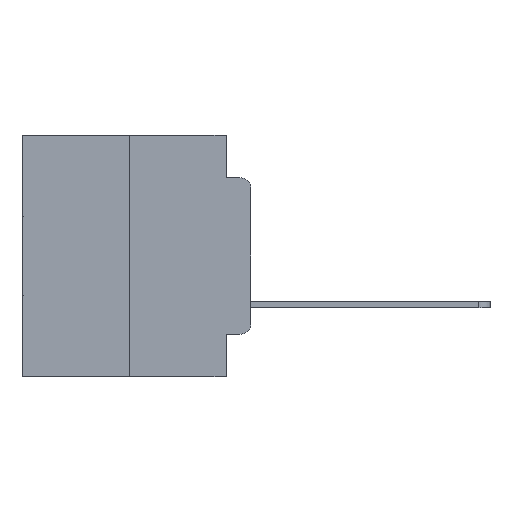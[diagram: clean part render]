
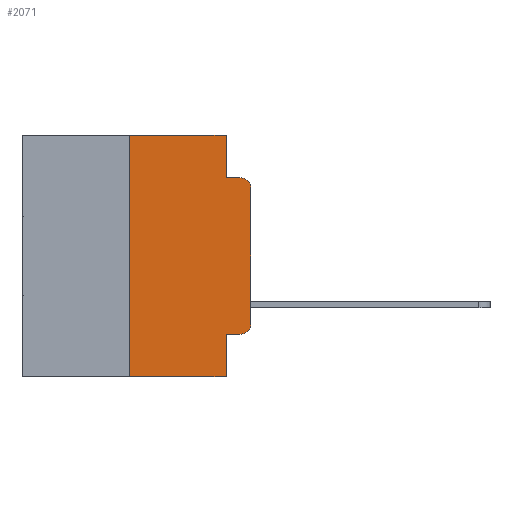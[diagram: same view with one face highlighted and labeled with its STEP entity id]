
A CAD part, left-side view. The second image highlights one B-rep face of the part: STEP entity #2071.
In plain terms, the highlighted planar face has unit normal (-1, 0, 0).
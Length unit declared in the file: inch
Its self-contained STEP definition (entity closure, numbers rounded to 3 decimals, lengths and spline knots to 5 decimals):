
#182 = DIRECTION ( 'NONE',  ( 0., 0., -1. ) ) ;
#361 = VECTOR ( 'NONE', #6799, 39.37008 ) ;
#924 = LINE ( 'NONE', #29368, #7049 ) ;
#1995 = VECTOR ( 'NONE', #3544, 39.37008 ) ;
#2071 = ADVANCED_FACE ( 'NONE', ( #7758 ), #21484, .F. ) ;
#2666 = VERTEX_POINT ( 'NONE', #7861 ) ;
#2777 = ORIENTED_EDGE ( 'NONE', *, *, #12554, .T. ) ;
#2829 = LINE ( 'NONE', #22086, #1995 ) ;
#3054 = VERTEX_POINT ( 'NONE', #5942 ) ;
#3544 = DIRECTION ( 'NONE',  ( 0., 0., -1. ) ) ;
#3761 = VERTEX_POINT ( 'NONE', #12208 ) ;
#4199 = CARTESIAN_POINT ( 'NONE',  ( 0., 0.051, -0.0885 ) ) ;
#4955 = DIRECTION ( 'NONE',  ( -1., 0., 0. ) ) ;
#5606 = ORIENTED_EDGE ( 'NONE', *, *, #14375, .T. ) ;
#5942 = CARTESIAN_POINT ( 'NONE',  ( 0., 0.02, -0.4115 ) ) ;
#6031 = AXIS2_PLACEMENT_3D ( 'NONE', #27563, #15197, #182 ) ;
#6092 = DIRECTION ( 'NONE',  ( 0., -1., 0. ) ) ;
#6799 = DIRECTION ( 'NONE',  ( 0., -1., 0. ) ) ;
#7049 = VECTOR ( 'NONE', #14979, 39.37008 ) ;
#7201 = ORIENTED_EDGE ( 'NONE', *, *, #12642, .F. ) ;
#7606 = VECTOR ( 'NONE', #6092, 39.37008 ) ;
#7656 = CARTESIAN_POINT ( 'NONE',  ( 0., 0., -0.3915 ) ) ;
#7758 = FACE_OUTER_BOUND ( 'NONE', #16010, .T. ) ;
#7861 = CARTESIAN_POINT ( 'NONE',  ( 0., 0.051, -0.0885 ) ) ;
#8324 = VECTOR ( 'NONE', #25672, 39.37008 ) ;
#8874 = LINE ( 'NONE', #10611, #9643 ) ;
#9643 = VECTOR ( 'NONE', #25686, 39.37008 ) ;
#9949 = VERTEX_POINT ( 'NONE', #19966 ) ;
#9962 = EDGE_CURVE ( 'NONE', #3761, #19557, #19168, .T. ) ;
#10521 = CIRCLE ( 'NONE', #6031, 0.02 ) ;
#10611 = CARTESIAN_POINT ( 'NONE',  ( 0., 0.051, -0.4115 ) ) ;
#11000 = CARTESIAN_POINT ( 'NONE',  ( 0., 0.25, 0. ) ) ;
#11378 = EDGE_CURVE ( 'NONE', #23673, #9949, #19353, .T. ) ;
#11418 = VERTEX_POINT ( 'NONE', #7656 ) ;
#11519 = EDGE_CURVE ( 'NONE', #3054, #11418, #10521, .T. ) ;
#12160 = ORIENTED_EDGE ( 'NONE', *, *, #11378, .T. ) ;
#12208 = CARTESIAN_POINT ( 'NONE',  ( 0., 0.25, -0.5 ) ) ;
#12554 = EDGE_CURVE ( 'NONE', #17698, #3054, #8874, .T. ) ;
#12642 = EDGE_CURVE ( 'NONE', #23695, #16998, #18239, .T. ) ;
#12915 = EDGE_CURVE ( 'NONE', #17698, #19557, #2829, .T. ) ;
#13374 = EDGE_CURVE ( 'NONE', #3761, #23695, #25785, .T. ) ;
#14375 = EDGE_CURVE ( 'NONE', #11418, #23673, #924, .T. ) ;
#14771 = CARTESIAN_POINT ( 'NONE',  ( 0., 0.473, 0. ) ) ;
#14979 = DIRECTION ( 'NONE',  ( 0., 0., 1. ) ) ;
#15027 = EDGE_CURVE ( 'NONE', #16998, #2666, #23178, .T. ) ;
#15197 = DIRECTION ( 'NONE',  ( -1., 0., 0. ) ) ;
#15631 = EDGE_CURVE ( 'NONE', #2666, #9949, #19604, .T. ) ;
#16010 = EDGE_LOOP ( 'NONE', ( #5606, #12160, #18180, #23668, #7201, #19492, #20140, #26148, #2777, #16510 ) ) ;
#16510 = ORIENTED_EDGE ( 'NONE', *, *, #11519, .T. ) ;
#16998 = VERTEX_POINT ( 'NONE', #21593 ) ;
#17554 = CARTESIAN_POINT ( 'NONE',  ( 0., 0.051, -0.5 ) ) ;
#17698 = VERTEX_POINT ( 'NONE', #19457 ) ;
#18180 = ORIENTED_EDGE ( 'NONE', *, *, #15631, .F. ) ;
#18239 = LINE ( 'NONE', #14771, #29015 ) ;
#19070 = CARTESIAN_POINT ( 'NONE',  ( 0., 0.02, -0.1085 ) ) ;
#19168 = LINE ( 'NONE', #27988, #7606 ) ;
#19353 = CIRCLE ( 'NONE', #24630, 0.02 ) ;
#19457 = CARTESIAN_POINT ( 'NONE',  ( 0., 0.051, -0.4115 ) ) ;
#19492 = ORIENTED_EDGE ( 'NONE', *, *, #13374, .F. ) ;
#19557 = VERTEX_POINT ( 'NONE', #17554 ) ;
#19604 = LINE ( 'NONE', #4199, #361 ) ;
#19966 = CARTESIAN_POINT ( 'NONE',  ( 0., 0.02, -0.0885 ) ) ;
#20140 = ORIENTED_EDGE ( 'NONE', *, *, #9962, .T. ) ;
#21156 = DIRECTION ( 'NONE',  ( 0., 0., -1. ) ) ;
#21420 = DIRECTION ( 'NONE',  ( 1., 0., 0. ) ) ;
#21455 = CARTESIAN_POINT ( 'NONE',  ( 0., 0.051, 0. ) ) ;
#21484 = PLANE ( 'NONE',  #23632 ) ;
#21593 = CARTESIAN_POINT ( 'NONE',  ( 0., 0.051, 0. ) ) ;
#21975 = CARTESIAN_POINT ( 'NONE',  ( 0., 0., -0.1085 ) ) ;
#21990 = DIRECTION ( 'NONE',  ( 0., 0., -1. ) ) ;
#22086 = CARTESIAN_POINT ( 'NONE',  ( 0., 0.051, 0. ) ) ;
#22551 = VECTOR ( 'NONE', #23518, 39.37008 ) ;
#22696 = CARTESIAN_POINT ( 'NONE',  ( 0., 0.473, 0. ) ) ;
#23175 = DIRECTION ( 'NONE',  ( 0., -1., 0. ) ) ;
#23178 = LINE ( 'NONE', #21455, #22551 ) ;
#23518 = DIRECTION ( 'NONE',  ( 0., 0., -1. ) ) ;
#23632 = AXIS2_PLACEMENT_3D ( 'NONE', #22696, #21420, #21990 ) ;
#23668 = ORIENTED_EDGE ( 'NONE', *, *, #15027, .F. ) ;
#23673 = VERTEX_POINT ( 'NONE', #21975 ) ;
#23674 = CARTESIAN_POINT ( 'NONE',  ( 0., 0.25, 0. ) ) ;
#23695 = VERTEX_POINT ( 'NONE', #11000 ) ;
#24630 = AXIS2_PLACEMENT_3D ( 'NONE', #19070, #4955, #21156 ) ;
#25672 = DIRECTION ( 'NONE',  ( 0., 0., 1. ) ) ;
#25686 = DIRECTION ( 'NONE',  ( 0., -1., 0. ) ) ;
#25785 = LINE ( 'NONE', #23674, #8324 ) ;
#26148 = ORIENTED_EDGE ( 'NONE', *, *, #12915, .F. ) ;
#27563 = CARTESIAN_POINT ( 'NONE',  ( 0., 0.02, -0.3915 ) ) ;
#27988 = CARTESIAN_POINT ( 'NONE',  ( 0., 0.473, -0.5 ) ) ;
#29015 = VECTOR ( 'NONE', #23175, 39.37008 ) ;
#29368 = CARTESIAN_POINT ( 'NONE',  ( 0., 0., 0. ) ) ;
